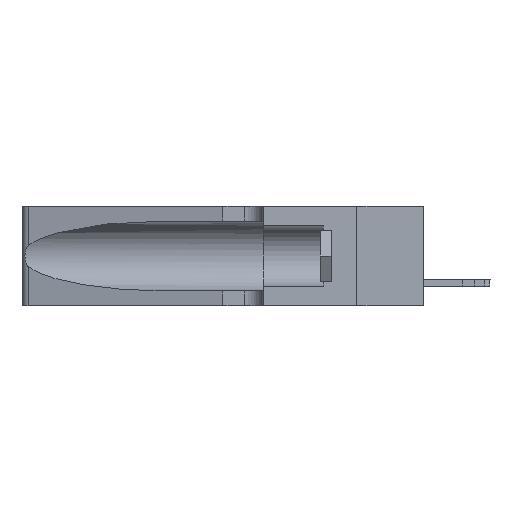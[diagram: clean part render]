
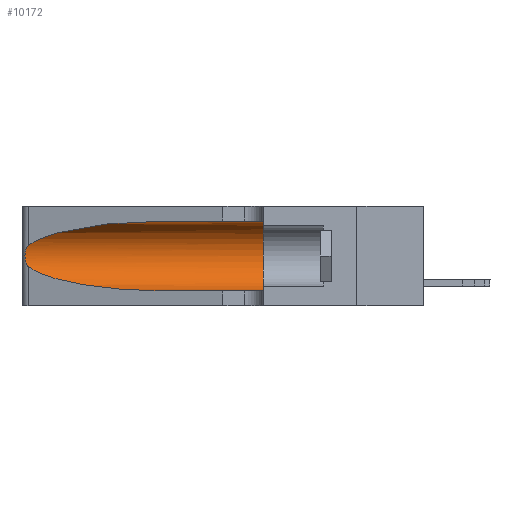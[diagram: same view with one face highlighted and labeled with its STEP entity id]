
A CAD part, left-side view. The second image highlights one B-rep face of the part: STEP entity #10172.
In plain terms, the highlighted cylindrical face has radius 3.308 mm (diameter 6.617 mm), a partial arc.
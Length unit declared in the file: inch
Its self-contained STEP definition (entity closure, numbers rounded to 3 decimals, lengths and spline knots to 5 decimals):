
#371 = ORIENTED_EDGE ( 'NONE', *, *, #13690, .F. ) ;
#982 = EDGE_CURVE ( 'NONE', #11197, #22863, #19209, .T. ) ;
#1037 = VERTEX_POINT ( 'NONE', #9973 ) ;
#1082 = FACE_OUTER_BOUND ( 'NONE', #6146, .T. ) ;
#1148 = VECTOR ( 'NONE', #19958, 39.37008 ) ;
#1442 = CARTESIAN_POINT ( 'NONE',  ( 0.1305, 1.61858, 0.05475 ) ) ;
#1488 = CARTESIAN_POINT ( 'NONE',  ( 0.25789, 1.23486, 0.15765 ) ) ;
#2262 = CARTESIAN_POINT ( 'NONE',  ( 0.1305, 1.61858, 0.31525 ) ) ;
#2363 = VECTOR ( 'NONE', #18521, 39.37008 ) ;
#2659 = LINE ( 'NONE', #2262, #2363 ) ;
#2723 = CARTESIAN_POINT ( 'NONE',  ( 0.2373, 1.15595, 0.28018 ) ) ;
#3261 = CARTESIAN_POINT ( 'NONE',  ( 0.25487, 1.22718, 0.14631 ) ) ;
#3330 = ORIENTED_EDGE ( 'NONE', *, *, #7389, .T. ) ;
#5336 = CARTESIAN_POINT ( 'NONE',  ( 0.26075, 1.23896, 0.19203 ) ) ;
#5384 = CYLINDRICAL_SURFACE ( 'NONE', #19777, 0.13025 ) ;
#5497 = CARTESIAN_POINT ( 'NONE',  ( 0.1305, 0.72297, 0.05475 ) ) ;
#5511 =( BOUNDED_CURVE ( )  B_SPLINE_CURVE ( 3, ( #20258, #7255, #10963, #5497 ),
 .UNSPECIFIED., .F., .T. ) 
 B_SPLINE_CURVE_WITH_KNOTS ( ( 4, 4 ),
 ( 3.44316, 4.71239 ),
 .UNSPECIFIED. ) 
 CURVE ( )  GEOMETRIC_REPRESENTATION_ITEM ( )  RATIONAL_B_SPLINE_CURVE ( ( 1., 0.87, 0.87, 1. ) ) 
 REPRESENTATION_ITEM ( '' )  );
#5542 = ORIENTED_EDGE ( 'NONE', *, *, #9121, .T. ) ;
#6146 = EDGE_LOOP ( 'NONE', ( #7239, #3330, #5542, #15699, #22003, #371 ) ) ;
#6835 = CARTESIAN_POINT ( 'NONE',  ( 0.25555, 1.22994, 0.2215 ) ) ;
#6876 = CARTESIAN_POINT ( 'NONE',  ( 0.1305, 1.61858, 0.185 ) ) ;
#6897 = VERTEX_POINT ( 'NONE', #18328 ) ;
#7094 = AXIS2_PLACEMENT_3D ( 'NONE', #15356, #21026, #10051 ) ;
#7239 = ORIENTED_EDGE ( 'NONE', *, *, #12010, .T. ) ;
#7255 = CARTESIAN_POINT ( 'NONE',  ( 0.2373, 1.15595, 0.08982 ) ) ;
#7389 = EDGE_CURVE ( 'NONE', #21255, #1037, #8011, .T. ) ;
#8011 = B_SPLINE_CURVE_WITH_KNOTS ( 'NONE', 3,
 ( #16260, #6835, #21607, #16342, #8932, #9014, #5336, #23777, #23460, #21776, #1488, #10547, #12401, #3261 ),
 .UNSPECIFIED., .F., .F.,
 ( 4, 2, 2, 2, 2, 2, 4 ),
 ( 0., 0.00027, 0.00053, 0.00107, 0.0016, 0.00187, 0.00214 ),
 .UNSPECIFIED. ) ;
#8535 = VERTEX_POINT ( 'NONE', #23081 ) ;
#8932 = CARTESIAN_POINT ( 'NONE',  ( 0.25854, 1.2359, 0.20912 ) ) ;
#9014 = CARTESIAN_POINT ( 'NONE',  ( 0.26018, 1.23835, 0.19895 ) ) ;
#9121 = EDGE_CURVE ( 'NONE', #1037, #6897, #5511, .T. ) ;
#9953 = CARTESIAN_POINT ( 'NONE',  ( 0.1305, 0.72297, 0.31525 ) ) ;
#9973 = CARTESIAN_POINT ( 'NONE',  ( 0.25487, 1.22718, 0.14631 ) ) ;
#10051 = DIRECTION ( 'NONE',  ( 0., 0., 1. ) ) ;
#10150 = CARTESIAN_POINT ( 'NONE',  ( 0.25487, 1.22718, 0.22369 ) ) ;
#10172 = ADVANCED_FACE ( 'NONE', ( #1082 ), #5384, .F. ) ;
#10547 = CARTESIAN_POINT ( 'NONE',  ( 0.25639, 1.23186, 0.15144 ) ) ;
#10963 = CARTESIAN_POINT ( 'NONE',  ( 0.18966, 0.96281, 0.05475 ) ) ;
#11197 = VERTEX_POINT ( 'NONE', #22893 ) ;
#12010 = EDGE_CURVE ( 'NONE', #8535, #21255, #14046, .T. ) ;
#12401 = CARTESIAN_POINT ( 'NONE',  ( 0.25555, 1.22993, 0.14849 ) ) ;
#13481 = CARTESIAN_POINT ( 'NONE',  ( 0.18966, 0.96281, 0.31525 ) ) ;
#13690 = EDGE_CURVE ( 'NONE', #8535, #11197, #2659, .T. ) ;
#14046 =( BOUNDED_CURVE ( )  B_SPLINE_CURVE ( 3, ( #9953, #13481, #2723, #17412 ),
 .UNSPECIFIED., .F., .F. ) 
 B_SPLINE_CURVE_WITH_KNOTS ( ( 4, 4 ),
 ( 1.5708, 2.84003 ),
 .UNSPECIFIED. ) 
 CURVE ( )  GEOMETRIC_REPRESENTATION_ITEM ( )  RATIONAL_B_SPLINE_CURVE ( ( 1., 0.87, 0.87, 1. ) ) 
 REPRESENTATION_ITEM ( '' )  );
#14908 = EDGE_CURVE ( 'NONE', #6897, #22863, #17238, .T. ) ;
#15356 = CARTESIAN_POINT ( 'NONE',  ( 0.1305, 0.35, 0.185 ) ) ;
#15699 = ORIENTED_EDGE ( 'NONE', *, *, #14908, .T. ) ;
#15749 = DIRECTION ( 'NONE',  ( 0., -1., 0. ) ) ;
#16260 = CARTESIAN_POINT ( 'NONE',  ( 0.25487, 1.22718, 0.22369 ) ) ;
#16342 = CARTESIAN_POINT ( 'NONE',  ( 0.25787, 1.23484, 0.2124 ) ) ;
#17238 = LINE ( 'NONE', #1442, #1148 ) ;
#17412 = CARTESIAN_POINT ( 'NONE',  ( 0.25487, 1.22718, 0.22369 ) ) ;
#18328 = CARTESIAN_POINT ( 'NONE',  ( 0.1305, 0.72297, 0.05475 ) ) ;
#18521 = DIRECTION ( 'NONE',  ( 0., -1., 0. ) ) ;
#19209 = CIRCLE ( 'NONE', #7094, 0.13025 ) ;
#19486 = DIRECTION ( 'NONE',  ( 0., 0., -1. ) ) ;
#19777 = AXIS2_PLACEMENT_3D ( 'NONE', #6876, #15749, #19486 ) ;
#19958 = DIRECTION ( 'NONE',  ( 0., -1., 0. ) ) ;
#20258 = CARTESIAN_POINT ( 'NONE',  ( 0.25487, 1.22718, 0.14631 ) ) ;
#20725 = CARTESIAN_POINT ( 'NONE',  ( 0.1305, 0.35, 0.05475 ) ) ;
#21026 = DIRECTION ( 'NONE',  ( 0., 1., 0. ) ) ;
#21255 = VERTEX_POINT ( 'NONE', #10150 ) ;
#21607 = CARTESIAN_POINT ( 'NONE',  ( 0.25639, 1.23184, 0.21858 ) ) ;
#21776 = CARTESIAN_POINT ( 'NONE',  ( 0.25856, 1.23593, 0.16098 ) ) ;
#22003 = ORIENTED_EDGE ( 'NONE', *, *, #982, .F. ) ;
#22863 = VERTEX_POINT ( 'NONE', #20725 ) ;
#22893 = CARTESIAN_POINT ( 'NONE',  ( 0.1305, 0.35, 0.31525 ) ) ;
#23081 = CARTESIAN_POINT ( 'NONE',  ( 0.1305, 0.72297, 0.31525 ) ) ;
#23460 = CARTESIAN_POINT ( 'NONE',  ( 0.26017, 1.23833, 0.17102 ) ) ;
#23777 = CARTESIAN_POINT ( 'NONE',  ( 0.26075, 1.23896, 0.178 ) ) ;
